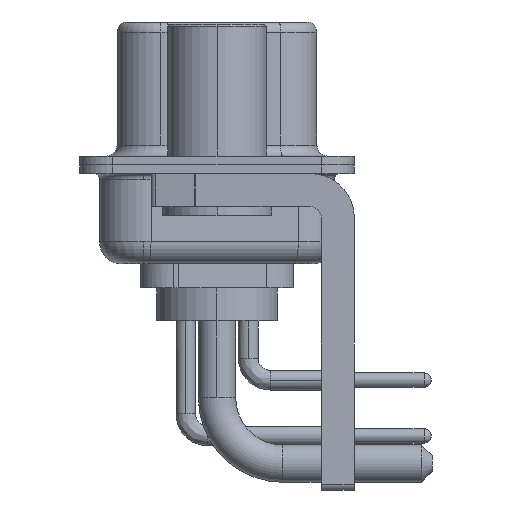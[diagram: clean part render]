
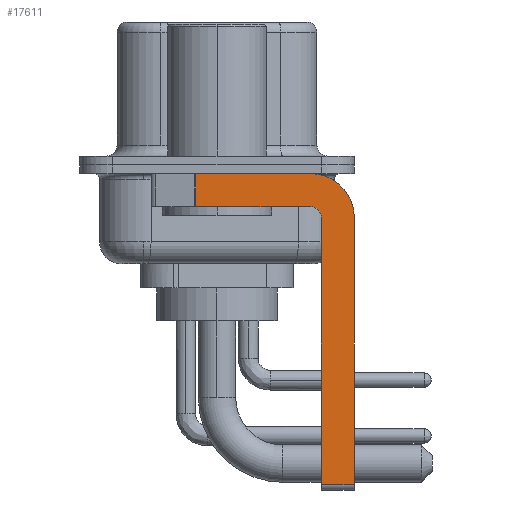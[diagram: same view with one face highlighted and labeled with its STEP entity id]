
A CAD part, left-side view. The second image highlights one B-rep face of the part: STEP entity #17611.
In plain terms, the highlighted planar face has unit normal (-1, 0, 0).
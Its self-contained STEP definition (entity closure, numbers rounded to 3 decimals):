
#647 = AXIS2_PLACEMENT_3D ( 'NONE', #9586, #14911, #14762 ) ;
#1700 = DIRECTION ( 'NONE',  ( 0., -1., 0. ) ) ;
#2452 = DIRECTION ( 'NONE',  ( 0., 0., 1. ) ) ;
#2496 = ORIENTED_EDGE ( 'NONE', *, *, #10453, .F. ) ;
#2535 = LINE ( 'NONE', #24061, #8651 ) ;
#2600 = VERTEX_POINT ( 'NONE', #4842 ) ;
#3066 = CARTESIAN_POINT ( 'NONE',  ( -2.9, 0.978, -0.4 ) ) ;
#3204 = DIRECTION ( 'NONE',  ( 0., -1., 0. ) ) ;
#3769 = ORIENTED_EDGE ( 'NONE', *, *, #5850, .F. ) ;
#4008 = LINE ( 'NONE', #30396, #13385 ) ;
#4842 = CARTESIAN_POINT ( 'NONE',  ( -2.9, 0.978, -1.9 ) ) ;
#5850 = EDGE_CURVE ( 'NONE', #15106, #26875, #22914, .T. ) ;
#6297 = VECTOR ( 'NONE', #1700, 1000. ) ;
#6629 = EDGE_CURVE ( 'NONE', #12466, #23952, #4008, .T. ) ;
#8651 = VECTOR ( 'NONE', #19038, 1000. ) ;
#8884 = DIRECTION ( 'NONE',  ( 0., 0., 1. ) ) ;
#9004 = CARTESIAN_POINT ( 'NONE',  ( -2.9, -4.25, -0.4 ) ) ;
#9586 = CARTESIAN_POINT ( 'NONE',  ( -2.9, -4.25, -2.4 ) ) ;
#9641 = CARTESIAN_POINT ( 'NONE',  ( -2.9, -6.25, -2.4 ) ) ;
#10012 = DIRECTION ( 'NONE',  ( 1., 0., 0. ) ) ;
#10228 = VERTEX_POINT ( 'NONE', #9641 ) ;
#10453 = EDGE_CURVE ( 'NONE', #23952, #18827, #25891, .T. ) ;
#10560 = AXIS2_PLACEMENT_3D ( 'NONE', #12366, #10012, #14404 ) ;
#11670 = CARTESIAN_POINT ( 'NONE',  ( -2.9, 0.978, -1.9 ) ) ;
#11945 = FACE_OUTER_BOUND ( 'NONE', #15863, .T. ) ;
#12073 = VERTEX_POINT ( 'NONE', #27713 ) ;
#12083 = CIRCLE ( 'NONE', #10560, 2. ) ;
#12366 = CARTESIAN_POINT ( 'NONE',  ( -2.9, -4.25, -2.4 ) ) ;
#12377 = AXIS2_PLACEMENT_3D ( 'NONE', #18796, #21787, #2452 ) ;
#12466 = VERTEX_POINT ( 'NONE', #22666 ) ;
#13385 = VECTOR ( 'NONE', #8884, 1000. ) ;
#14045 = EDGE_CURVE ( 'NONE', #15106, #2600, #17006, .T. ) ;
#14404 = DIRECTION ( 'NONE',  ( 0., 0., -1. ) ) ;
#14652 = VECTOR ( 'NONE', #3204, 1000. ) ;
#14762 = DIRECTION ( 'NONE',  ( 0., 0., -1. ) ) ;
#14911 = DIRECTION ( 'NONE',  ( 1., 0., 0. ) ) ;
#15106 = VERTEX_POINT ( 'NONE', #3066 ) ;
#15758 = CARTESIAN_POINT ( 'NONE',  ( -2.9, -4.25, -1.9 ) ) ;
#15863 = EDGE_LOOP ( 'NONE', ( #3769, #27198, #22806, #2496, #28952, #16464, #26384, #17485 ) ) ;
#16464 = ORIENTED_EDGE ( 'NONE', *, *, #21527, .T. ) ;
#16470 = CARTESIAN_POINT ( 'NONE',  ( -2.9, -4.25, -1.9 ) ) ;
#16608 = VECTOR ( 'NONE', #21560, 1000. ) ;
#17006 = LINE ( 'NONE', #11670, #16608 ) ;
#17062 = CARTESIAN_POINT ( 'NONE',  ( -2.9, -4.75, -2.4 ) ) ;
#17097 = EDGE_CURVE ( 'NONE', #10228, #12073, #2535, .T. ) ;
#17485 = ORIENTED_EDGE ( 'NONE', *, *, #26038, .F. ) ;
#17611 = ADVANCED_FACE ( 'NONE', ( #11945 ), #21523, .F. ) ;
#17974 = LINE ( 'NONE', #25177, #14652 ) ;
#18796 = CARTESIAN_POINT ( 'NONE',  ( -2.9, -4.25, -2.4 ) ) ;
#18827 = VERTEX_POINT ( 'NONE', #15758 ) ;
#19038 = DIRECTION ( 'NONE',  ( 0., 0., -1. ) ) ;
#21523 = PLANE ( 'NONE',  #647 ) ;
#21527 = EDGE_CURVE ( 'NONE', #12466, #12073, #17974, .T. ) ;
#21560 = DIRECTION ( 'NONE',  ( 0., 0., -1. ) ) ;
#21787 = DIRECTION ( 'NONE',  ( -1., 0., 0. ) ) ;
#22666 = CARTESIAN_POINT ( 'NONE',  ( -2.9, -4.75, -14.55 ) ) ;
#22806 = ORIENTED_EDGE ( 'NONE', *, *, #30649, .F. ) ;
#22914 = LINE ( 'NONE', #25115, #6297 ) ;
#23533 = DIRECTION ( 'NONE',  ( 0., 1., 0. ) ) ;
#23952 = VERTEX_POINT ( 'NONE', #17062 ) ;
#24061 = CARTESIAN_POINT ( 'NONE',  ( -2.9, -6.25, -2.4 ) ) ;
#25115 = CARTESIAN_POINT ( 'NONE',  ( -2.9, 3., -0.4 ) ) ;
#25177 = CARTESIAN_POINT ( 'NONE',  ( -2.9, -4.25, -14.55 ) ) ;
#25891 = CIRCLE ( 'NONE', #12377, 0.5 ) ;
#26038 = EDGE_CURVE ( 'NONE', #26875, #10228, #12083, .T. ) ;
#26384 = ORIENTED_EDGE ( 'NONE', *, *, #17097, .F. ) ;
#26493 = VECTOR ( 'NONE', #23533, 1000. ) ;
#26875 = VERTEX_POINT ( 'NONE', #9004 ) ;
#27198 = ORIENTED_EDGE ( 'NONE', *, *, #14045, .T. ) ;
#27713 = CARTESIAN_POINT ( 'NONE',  ( -2.9, -6.25, -14.55 ) ) ;
#28232 = LINE ( 'NONE', #16470, #26493 ) ;
#28952 = ORIENTED_EDGE ( 'NONE', *, *, #6629, .F. ) ;
#30396 = CARTESIAN_POINT ( 'NONE',  ( -2.9, -4.75, -14.8 ) ) ;
#30649 = EDGE_CURVE ( 'NONE', #18827, #2600, #28232, .T. ) ;
